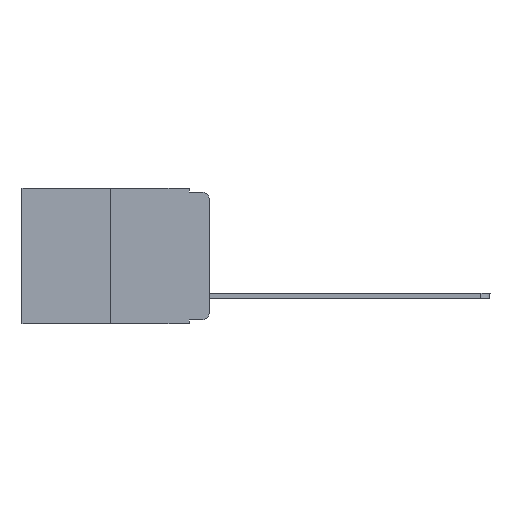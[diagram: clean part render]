
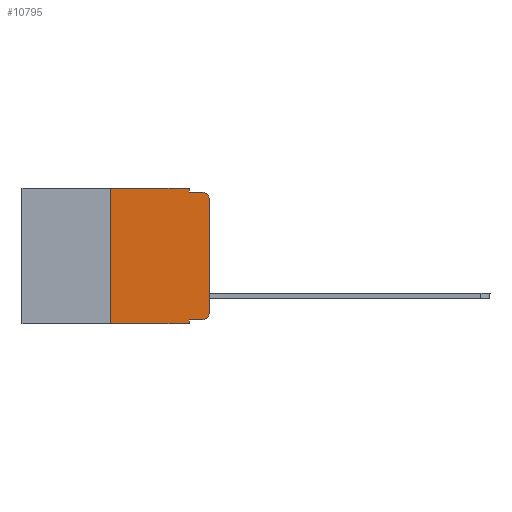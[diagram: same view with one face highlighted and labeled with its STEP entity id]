
A CAD part, left-side view. The second image highlights one B-rep face of the part: STEP entity #10795.
In plain terms, the highlighted planar face has unit normal (-1, 0, 0).
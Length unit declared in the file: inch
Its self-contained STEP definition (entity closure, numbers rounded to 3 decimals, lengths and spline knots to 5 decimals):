
#29 = CARTESIAN_POINT ( 'NONE',  ( 0., 0.25, 0. ) ) ;
#35 = VECTOR ( 'NONE', #6843, 39.37008 ) ;
#212 = DIRECTION ( 'NONE',  ( 0., -1., 0. ) ) ;
#341 = EDGE_LOOP ( 'NONE', ( #9690, #6126, #7227, #11032, #12349, #11912, #4929, #13186, #1193, #10125 ) ) ;
#356 = DIRECTION ( 'NONE',  ( 0., 0., 1. ) ) ;
#509 = EDGE_CURVE ( 'NONE', #11397, #9557, #1721, .T. ) ;
#529 = CARTESIAN_POINT ( 'NONE',  ( 0., 0., -0.03 ) ) ;
#680 = DIRECTION ( 'NONE',  ( -1., 0., 0. ) ) ;
#828 = DIRECTION ( 'NONE',  ( 0., 0., -1. ) ) ;
#985 = CIRCLE ( 'NONE', #4693, 0.02 ) ;
#1068 = VERTEX_POINT ( 'NONE', #29 ) ;
#1193 = ORIENTED_EDGE ( 'NONE', *, *, #9222, .T. ) ;
#1260 = LINE ( 'NONE', #2651, #14417 ) ;
#1390 = EDGE_CURVE ( 'NONE', #7784, #10211, #985, .T. ) ;
#1401 = CARTESIAN_POINT ( 'NONE',  ( 0., 0.02, -0.333 ) ) ;
#1721 = LINE ( 'NONE', #7568, #3965 ) ;
#2125 = VERTEX_POINT ( 'NONE', #9174 ) ;
#2600 = EDGE_CURVE ( 'NONE', #8955, #9294, #7399, .T. ) ;
#2651 = CARTESIAN_POINT ( 'NONE',  ( 0., 0.25, 0. ) ) ;
#3012 = CARTESIAN_POINT ( 'NONE',  ( 0., 0.051, -0.333 ) ) ;
#3591 = DIRECTION ( 'NONE',  ( 0., 0., 1. ) ) ;
#3612 = EDGE_CURVE ( 'NONE', #10817, #9294, #10046, .T. ) ;
#3616 = VECTOR ( 'NONE', #356, 39.37008 ) ;
#3965 = VECTOR ( 'NONE', #8507, 39.37008 ) ;
#4113 = DIRECTION ( 'NONE',  ( 0., -1., 0. ) ) ;
#4335 = CARTESIAN_POINT ( 'NONE',  ( 0., 0.051, -0.343 ) ) ;
#4693 = AXIS2_PLACEMENT_3D ( 'NONE', #10810, #6076, #828 ) ;
#4929 = ORIENTED_EDGE ( 'NONE', *, *, #2600, .T. ) ;
#5107 = DIRECTION ( 'NONE',  ( 0., 0., -1. ) ) ;
#5195 = LINE ( 'NONE', #3012, #10723 ) ;
#5400 = AXIS2_PLACEMENT_3D ( 'NONE', #10655, #680, #5107 ) ;
#5430 = CARTESIAN_POINT ( 'NONE',  ( 0., 0.02, -0.01 ) ) ;
#5748 = CARTESIAN_POINT ( 'NONE',  ( 0., 0.051, -0.01 ) ) ;
#5936 = FACE_OUTER_BOUND ( 'NONE', #341, .T. ) ;
#6076 = DIRECTION ( 'NONE',  ( -1., 0., 0. ) ) ;
#6126 = ORIENTED_EDGE ( 'NONE', *, *, #1390, .T. ) ;
#6131 = CARTESIAN_POINT ( 'NONE',  ( 0., 0.051, 0. ) ) ;
#6293 = EDGE_CURVE ( 'NONE', #8955, #1068, #1260, .T. ) ;
#6843 = DIRECTION ( 'NONE',  ( 0., -1., 0. ) ) ;
#6885 = CARTESIAN_POINT ( 'NONE',  ( 0., 0.051, -0.333 ) ) ;
#6959 = PLANE ( 'NONE',  #8895 ) ;
#7031 = DIRECTION ( 'NONE',  ( 0., 0., -1. ) ) ;
#7198 = CARTESIAN_POINT ( 'NONE',  ( 0., 0., 0. ) ) ;
#7227 = ORIENTED_EDGE ( 'NONE', *, *, #7280, .F. ) ;
#7280 = EDGE_CURVE ( 'NONE', #9557, #10211, #11296, .T. ) ;
#7399 = LINE ( 'NONE', #8397, #10408 ) ;
#7568 = CARTESIAN_POINT ( 'NONE',  ( 0., 0.051, 0. ) ) ;
#7784 = VERTEX_POINT ( 'NONE', #529 ) ;
#8397 = CARTESIAN_POINT ( 'NONE',  ( 0., 0.473, -0.343 ) ) ;
#8434 = CIRCLE ( 'NONE', #5400, 0.02 ) ;
#8471 = EDGE_CURVE ( 'NONE', #1068, #11397, #13265, .T. ) ;
#8507 = DIRECTION ( 'NONE',  ( 0., 0., -1. ) ) ;
#8749 = CARTESIAN_POINT ( 'NONE',  ( 0., 0.051, 0. ) ) ;
#8895 = AXIS2_PLACEMENT_3D ( 'NONE', #10514, #12423, #7031 ) ;
#8955 = VERTEX_POINT ( 'NONE', #11192 ) ;
#9174 = CARTESIAN_POINT ( 'NONE',  ( 0., 0., -0.313 ) ) ;
#9222 = EDGE_CURVE ( 'NONE', #10817, #10763, #5195, .T. ) ;
#9294 = VERTEX_POINT ( 'NONE', #4335 ) ;
#9331 = VECTOR ( 'NONE', #212, 39.37008 ) ;
#9557 = VERTEX_POINT ( 'NONE', #10489 ) ;
#9690 = ORIENTED_EDGE ( 'NONE', *, *, #14182, .T. ) ;
#10046 = LINE ( 'NONE', #8749, #13887 ) ;
#10125 = ORIENTED_EDGE ( 'NONE', *, *, #11009, .T. ) ;
#10211 = VERTEX_POINT ( 'NONE', #5430 ) ;
#10408 = VECTOR ( 'NONE', #13894, 39.37008 ) ;
#10489 = CARTESIAN_POINT ( 'NONE',  ( 0., 0.051, -0.01 ) ) ;
#10514 = CARTESIAN_POINT ( 'NONE',  ( 0., 0.473, 0. ) ) ;
#10655 = CARTESIAN_POINT ( 'NONE',  ( 0., 0.02, -0.313 ) ) ;
#10723 = VECTOR ( 'NONE', #4113, 39.37008 ) ;
#10763 = VERTEX_POINT ( 'NONE', #1401 ) ;
#10795 = ADVANCED_FACE ( 'NONE', ( #5936 ), #6959, .F. ) ;
#10810 = CARTESIAN_POINT ( 'NONE',  ( 0., 0.02, -0.03 ) ) ;
#10817 = VERTEX_POINT ( 'NONE', #6885 ) ;
#11009 = EDGE_CURVE ( 'NONE', #10763, #2125, #8434, .T. ) ;
#11032 = ORIENTED_EDGE ( 'NONE', *, *, #509, .F. ) ;
#11192 = CARTESIAN_POINT ( 'NONE',  ( 0., 0.25, -0.343 ) ) ;
#11210 = CARTESIAN_POINT ( 'NONE',  ( 0., 0.473, 0. ) ) ;
#11296 = LINE ( 'NONE', #5748, #9331 ) ;
#11397 = VERTEX_POINT ( 'NONE', #6131 ) ;
#11912 = ORIENTED_EDGE ( 'NONE', *, *, #6293, .F. ) ;
#12349 = ORIENTED_EDGE ( 'NONE', *, *, #8471, .F. ) ;
#12423 = DIRECTION ( 'NONE',  ( 1., 0., 0. ) ) ;
#13186 = ORIENTED_EDGE ( 'NONE', *, *, #3612, .F. ) ;
#13213 = DIRECTION ( 'NONE',  ( 0., 0., -1. ) ) ;
#13265 = LINE ( 'NONE', #11210, #35 ) ;
#13841 = LINE ( 'NONE', #7198, #3616 ) ;
#13887 = VECTOR ( 'NONE', #13213, 39.37008 ) ;
#13894 = DIRECTION ( 'NONE',  ( 0., -1., 0. ) ) ;
#14182 = EDGE_CURVE ( 'NONE', #2125, #7784, #13841, .T. ) ;
#14417 = VECTOR ( 'NONE', #3591, 39.37008 ) ;
